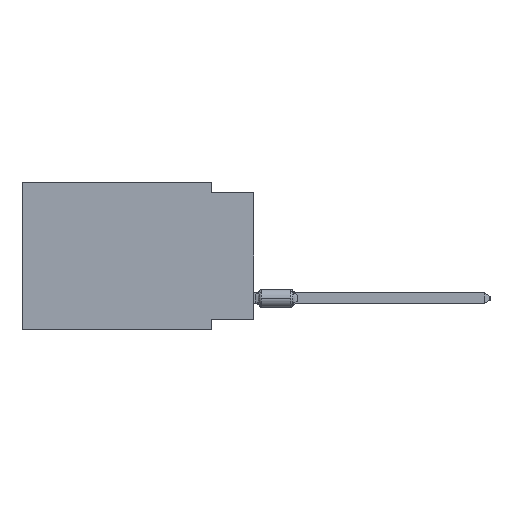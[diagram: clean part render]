
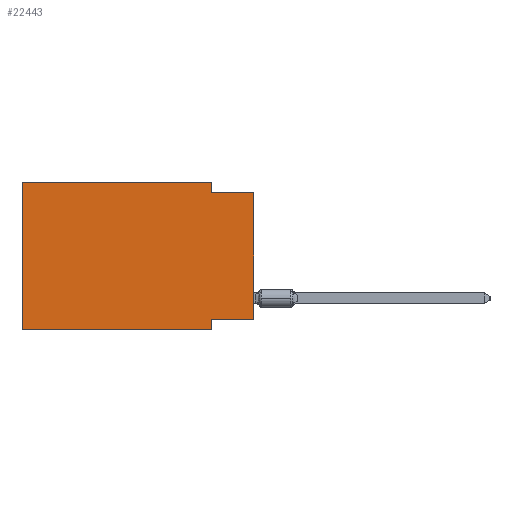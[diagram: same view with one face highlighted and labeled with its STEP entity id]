
A CAD part, left-side view. The second image highlights one B-rep face of the part: STEP entity #22443.
In plain terms, the highlighted planar face has unit normal (-1, 0, 0).
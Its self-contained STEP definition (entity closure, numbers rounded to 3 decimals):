
#1357 = ORIENTED_EDGE ( 'NONE', *, *, #88137, .T. ) ;
#2917 = EDGE_LOOP ( 'NONE', ( #1357, #55021, #34103, #79897, #75906, #88885, #50542, #58132 ) ) ;
#5219 = LINE ( 'NONE', #94124, #93135 ) ;
#6946 = EDGE_CURVE ( 'NONE', #17958, #12219, #52473, .T. ) ;
#10015 = CARTESIAN_POINT ( 'NONE',  ( 0., 0., 0. ) ) ;
#10270 = CARTESIAN_POINT ( 'NONE',  ( 0., 13.97, 0. ) ) ;
#12219 = VERTEX_POINT ( 'NONE', #50010 ) ;
#13798 = CARTESIAN_POINT ( 'NONE',  ( 0., 0., -0.635 ) ) ;
#17958 = VERTEX_POINT ( 'NONE', #74732 ) ;
#20357 = CARTESIAN_POINT ( 'NONE',  ( 0., 2.54, -0.635 ) ) ;
#20458 = VERTEX_POINT ( 'NONE', #20357 ) ;
#21664 = VECTOR ( 'NONE', #23123, 1000. ) ;
#22443 = ADVANCED_FACE ( 'NONE', ( #59017 ), #60465, .F. ) ;
#22867 = DIRECTION ( 'NONE',  ( 0., 0., -1. ) ) ;
#22984 = VECTOR ( 'NONE', #32473, 1000. ) ;
#23123 = DIRECTION ( 'NONE',  ( 0., -1., 0. ) ) ;
#24472 = LINE ( 'NONE', #10270, #47602 ) ;
#25205 = EDGE_CURVE ( 'NONE', #17958, #32494, #84177, .T. ) ;
#25276 = VERTEX_POINT ( 'NONE', #80661 ) ;
#25805 = CARTESIAN_POINT ( 'NONE',  ( 0., 2.54, 0. ) ) ;
#31865 = CARTESIAN_POINT ( 'NONE',  ( 0., 2.54, -8.89 ) ) ;
#32473 = DIRECTION ( 'NONE',  ( 0., 0., 1. ) ) ;
#32494 = VERTEX_POINT ( 'NONE', #91048 ) ;
#33414 = CARTESIAN_POINT ( 'NONE',  ( 0., 2.54, 0. ) ) ;
#34085 = LINE ( 'NONE', #25805, #46938 ) ;
#34103 = ORIENTED_EDGE ( 'NONE', *, *, #37847, .F. ) ;
#34520 = DIRECTION ( 'NONE',  ( 0., 1., 0. ) ) ;
#36971 = VECTOR ( 'NONE', #70448, 1000. ) ;
#37847 = EDGE_CURVE ( 'NONE', #58817, #20458, #34085, .T. ) ;
#39187 = VECTOR ( 'NONE', #61633, 1000. ) ;
#39358 = VERTEX_POINT ( 'NONE', #13798 ) ;
#43647 = LINE ( 'NONE', #52423, #21664 ) ;
#45154 = CARTESIAN_POINT ( 'NONE',  ( 0., 13.97, 0. ) ) ;
#45453 = EDGE_CURVE ( 'NONE', #12219, #58817, #24472, .T. ) ;
#46184 = LINE ( 'NONE', #10015, #22984 ) ;
#46938 = VECTOR ( 'NONE', #63875, 1000. ) ;
#47602 = VECTOR ( 'NONE', #54253, 1000. ) ;
#50010 = CARTESIAN_POINT ( 'NONE',  ( 0., 13.97, 0. ) ) ;
#50542 = ORIENTED_EDGE ( 'NONE', *, *, #87259, .F. ) ;
#52423 = CARTESIAN_POINT ( 'NONE',  ( 0., 0., -0.635 ) ) ;
#52473 = LINE ( 'NONE', #45154, #75210 ) ;
#54253 = DIRECTION ( 'NONE',  ( 0., -1., 0. ) ) ;
#55021 = ORIENTED_EDGE ( 'NONE', *, *, #89654, .F. ) ;
#57791 = EDGE_CURVE ( 'NONE', #25276, #84552, #5219, .T. ) ;
#58132 = ORIENTED_EDGE ( 'NONE', *, *, #57791, .F. ) ;
#58531 = DIRECTION ( 'NONE',  ( 1., 0., 0. ) ) ;
#58817 = VERTEX_POINT ( 'NONE', #33414 ) ;
#59017 = FACE_OUTER_BOUND ( 'NONE', #2917, .T. ) ;
#59977 = CARTESIAN_POINT ( 'NONE',  ( 0., 13.97, 0. ) ) ;
#60465 = PLANE ( 'NONE',  #71118 ) ;
#61633 = DIRECTION ( 'NONE',  ( 0., 0., -1. ) ) ;
#62096 = LINE ( 'NONE', #31865, #39187 ) ;
#63875 = DIRECTION ( 'NONE',  ( 0., 0., -1. ) ) ;
#70448 = DIRECTION ( 'NONE',  ( 0., -1., 0. ) ) ;
#71118 = AXIS2_PLACEMENT_3D ( 'NONE', #59977, #58531, #22867 ) ;
#74732 = CARTESIAN_POINT ( 'NONE',  ( 0., 13.97, -8.89 ) ) ;
#75210 = VECTOR ( 'NONE', #75433, 1000. ) ;
#75433 = DIRECTION ( 'NONE',  ( 0., 0., 1. ) ) ;
#75906 = ORIENTED_EDGE ( 'NONE', *, *, #6946, .F. ) ;
#76852 = CARTESIAN_POINT ( 'NONE',  ( 0., 13.97, -8.89 ) ) ;
#79897 = ORIENTED_EDGE ( 'NONE', *, *, #45453, .F. ) ;
#80661 = CARTESIAN_POINT ( 'NONE',  ( 0., 0., -8.255 ) ) ;
#84177 = LINE ( 'NONE', #76852, #36971 ) ;
#84552 = VERTEX_POINT ( 'NONE', #95364 ) ;
#87259 = EDGE_CURVE ( 'NONE', #84552, #32494, #62096, .T. ) ;
#88137 = EDGE_CURVE ( 'NONE', #25276, #39358, #46184, .T. ) ;
#88885 = ORIENTED_EDGE ( 'NONE', *, *, #25205, .T. ) ;
#89654 = EDGE_CURVE ( 'NONE', #20458, #39358, #43647, .T. ) ;
#91048 = CARTESIAN_POINT ( 'NONE',  ( 0., 2.54, -8.89 ) ) ;
#93135 = VECTOR ( 'NONE', #34520, 1000. ) ;
#94124 = CARTESIAN_POINT ( 'NONE',  ( 0., 0., -8.255 ) ) ;
#95364 = CARTESIAN_POINT ( 'NONE',  ( 0., 2.54, -8.255 ) ) ;
